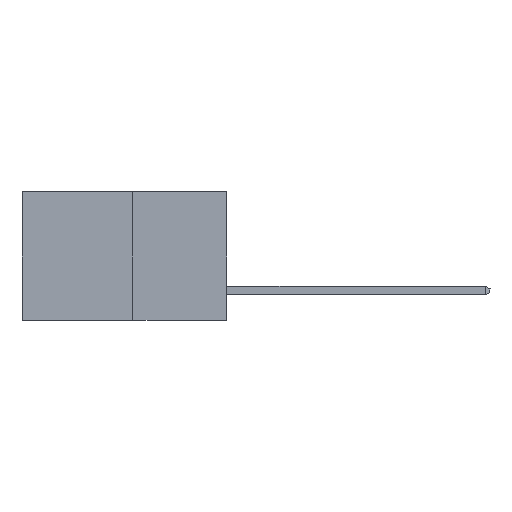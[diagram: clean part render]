
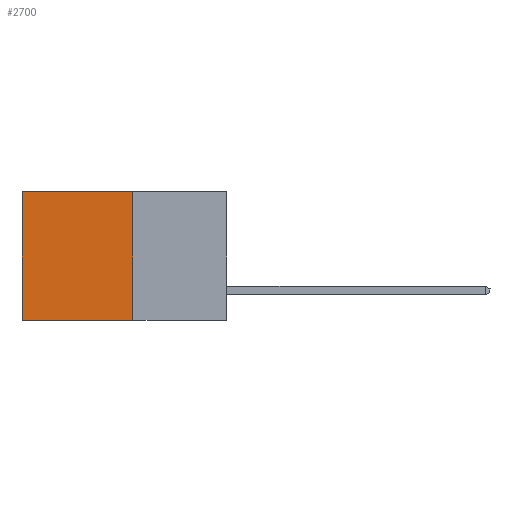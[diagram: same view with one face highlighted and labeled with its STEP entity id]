
A CAD part, left-side view. The second image highlights one B-rep face of the part: STEP entity #2700.
In plain terms, the highlighted planar face has unit normal (-1, 0, 0).
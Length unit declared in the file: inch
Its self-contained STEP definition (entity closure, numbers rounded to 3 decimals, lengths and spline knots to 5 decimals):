
#80 = ORIENTED_EDGE ( 'NONE', *, *, #5235, .T. ) ;
#796 = CARTESIAN_POINT ( 'NONE',  ( 0.277, 0.59, -0.37 ) ) ;
#1024 = CARTESIAN_POINT ( 'NONE',  ( 0.277, 0.27, -0.37 ) ) ;
#1091 = DIRECTION ( 'NONE',  ( 0., 0., -1. ) ) ;
#1305 = VECTOR ( 'NONE', #7339, 39.37008 ) ;
#1571 = VECTOR ( 'NONE', #1091, 39.37008 ) ;
#2495 = AXIS2_PLACEMENT_3D ( 'NONE', #3802, #2549, #4530 ) ;
#2549 = DIRECTION ( 'NONE',  ( 1., 0., 0. ) ) ;
#2700 = ADVANCED_FACE ( 'NONE', ( #2891 ), #4499, .F. ) ;
#2891 = FACE_OUTER_BOUND ( 'NONE', #5894, .T. ) ;
#2934 = VERTEX_POINT ( 'NONE', #7327 ) ;
#3802 = CARTESIAN_POINT ( 'NONE',  ( 0.277, 0.27, -0.37 ) ) ;
#3837 = EDGE_CURVE ( 'NONE', #7886, #2934, #10765, .T. ) ;
#3952 = LINE ( 'NONE', #14252, #7059 ) ;
#4185 = ORIENTED_EDGE ( 'NONE', *, *, #6739, .F. ) ;
#4372 = VERTEX_POINT ( 'NONE', #796 ) ;
#4442 = LINE ( 'NONE', #7335, #1305 ) ;
#4499 = PLANE ( 'NONE',  #2495 ) ;
#4530 = DIRECTION ( 'NONE',  ( 0., 0., -1. ) ) ;
#5019 = ORIENTED_EDGE ( 'NONE', *, *, #13869, .T. ) ;
#5182 = DIRECTION ( 'NONE',  ( 0., 1., 0. ) ) ;
#5235 = EDGE_CURVE ( 'NONE', #8986, #4372, #3952, .T. ) ;
#5894 = EDGE_LOOP ( 'NONE', ( #80, #4185, #10714, #5019 ) ) ;
#6739 = EDGE_CURVE ( 'NONE', #2934, #4372, #4442, .T. ) ;
#7059 = VECTOR ( 'NONE', #14434, 39.37008 ) ;
#7327 = CARTESIAN_POINT ( 'NONE',  ( 0.277, 0.27, -0.37 ) ) ;
#7335 = CARTESIAN_POINT ( 'NONE',  ( 0.277, 0.27, -0.37 ) ) ;
#7339 = DIRECTION ( 'NONE',  ( 0., 1., 0. ) ) ;
#7886 = VERTEX_POINT ( 'NONE', #8213 ) ;
#8213 = CARTESIAN_POINT ( 'NONE',  ( 0.277, 0.27, 0. ) ) ;
#8986 = VERTEX_POINT ( 'NONE', #14865 ) ;
#10562 = LINE ( 'NONE', #11986, #13579 ) ;
#10714 = ORIENTED_EDGE ( 'NONE', *, *, #3837, .F. ) ;
#10765 = LINE ( 'NONE', #1024, #1571 ) ;
#11986 = CARTESIAN_POINT ( 'NONE',  ( 0.277, 0.27, 0. ) ) ;
#13579 = VECTOR ( 'NONE', #5182, 39.37008 ) ;
#13869 = EDGE_CURVE ( 'NONE', #7886, #8986, #10562, .T. ) ;
#14252 = CARTESIAN_POINT ( 'NONE',  ( 0.277, 0.59, -0.37 ) ) ;
#14434 = DIRECTION ( 'NONE',  ( 0., 0., -1. ) ) ;
#14865 = CARTESIAN_POINT ( 'NONE',  ( 0.277, 0.59, 0. ) ) ;
